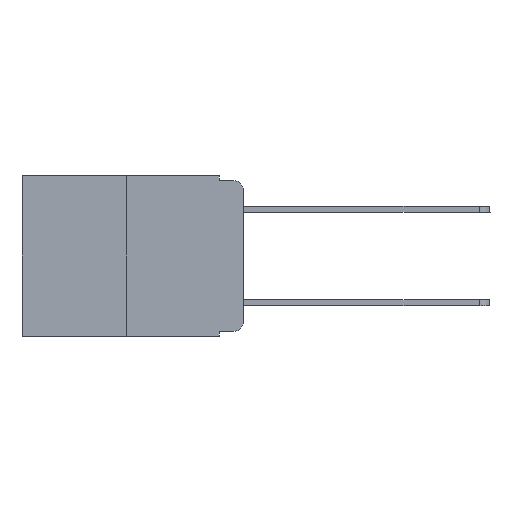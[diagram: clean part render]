
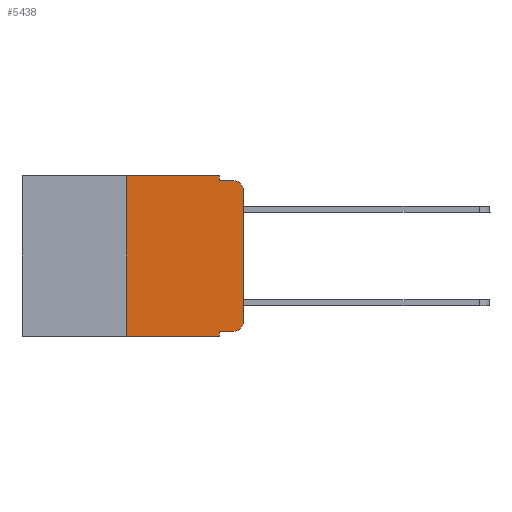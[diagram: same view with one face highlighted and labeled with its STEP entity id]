
A CAD part, left-side view. The second image highlights one B-rep face of the part: STEP entity #5438.
In plain terms, the highlighted planar face has unit normal (-1, 0, 0).
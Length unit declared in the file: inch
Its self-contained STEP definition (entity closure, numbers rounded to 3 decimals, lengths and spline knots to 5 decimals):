
#34 = CARTESIAN_POINT ( 'NONE',  ( 0., 0.25, -0.343 ) ) ;
#55 = EDGE_CURVE ( 'NONE', #1467, #11589, #5003, .T. ) ;
#94 = ORIENTED_EDGE ( 'NONE', *, *, #7449, .T. ) ;
#818 = LINE ( 'NONE', #9619, #1264 ) ;
#822 = CARTESIAN_POINT ( 'NONE',  ( 0., 0.473, 0. ) ) ;
#909 = ORIENTED_EDGE ( 'NONE', *, *, #7644, .T. ) ;
#1184 = LINE ( 'NONE', #5515, #7079 ) ;
#1203 = LINE ( 'NONE', #2210, #11564 ) ;
#1264 = VECTOR ( 'NONE', #2092, 39.37008 ) ;
#1420 = AXIS2_PLACEMENT_3D ( 'NONE', #4175, #13900, #6305 ) ;
#1427 = EDGE_CURVE ( 'NONE', #5306, #13583, #5239, .T. ) ;
#1467 = VERTEX_POINT ( 'NONE', #11957 ) ;
#1796 = DIRECTION ( 'NONE',  ( 0., 0., -1. ) ) ;
#1996 = VECTOR ( 'NONE', #12191, 39.37008 ) ;
#2050 = DIRECTION ( 'NONE',  ( 0., 0., -1. ) ) ;
#2092 = DIRECTION ( 'NONE',  ( 0., -1., 0. ) ) ;
#2210 = CARTESIAN_POINT ( 'NONE',  ( 0., 0., 0. ) ) ;
#2395 = EDGE_CURVE ( 'NONE', #11589, #13583, #818, .T. ) ;
#2417 = EDGE_LOOP ( 'NONE', ( #6809, #4321, #7530, #4868, #9445, #11373, #909, #8463, #12309, #94 ) ) ;
#2579 = VERTEX_POINT ( 'NONE', #34 ) ;
#3213 = CARTESIAN_POINT ( 'NONE',  ( 0., 0., -0.313 ) ) ;
#3253 = VERTEX_POINT ( 'NONE', #3801 ) ;
#3503 = CARTESIAN_POINT ( 'NONE',  ( 0., 0., -0.03 ) ) ;
#3801 = CARTESIAN_POINT ( 'NONE',  ( 0., 0.051, -0.333 ) ) ;
#4073 = EDGE_CURVE ( 'NONE', #3253, #7361, #7893, .T. ) ;
#4175 = CARTESIAN_POINT ( 'NONE',  ( 0., 0.02, -0.313 ) ) ;
#4321 = ORIENTED_EDGE ( 'NONE', *, *, #1427, .T. ) ;
#4738 = CARTESIAN_POINT ( 'NONE',  ( 0., 0.051, -0.333 ) ) ;
#4868 = ORIENTED_EDGE ( 'NONE', *, *, #55, .F. ) ;
#5003 = LINE ( 'NONE', #10753, #5395 ) ;
#5228 = DIRECTION ( 'NONE',  ( -1., 0., 0. ) ) ;
#5239 = CIRCLE ( 'NONE', #12024, 0.02 ) ;
#5306 = VERTEX_POINT ( 'NONE', #3503 ) ;
#5395 = VECTOR ( 'NONE', #13682, 39.37008 ) ;
#5438 = ADVANCED_FACE ( 'NONE', ( #8261 ), #10230, .F. ) ;
#5470 = AXIS2_PLACEMENT_3D ( 'NONE', #822, #6115, #8333 ) ;
#5472 = EDGE_CURVE ( 'NONE', #3253, #13927, #11492, .T. ) ;
#5515 = CARTESIAN_POINT ( 'NONE',  ( 0., 0.25, 0. ) ) ;
#5530 = DIRECTION ( 'NONE',  ( 0., -1., 0. ) ) ;
#5655 = LINE ( 'NONE', #12161, #10930 ) ;
#5964 = EDGE_CURVE ( 'NONE', #12203, #5306, #1203, .T. ) ;
#6115 = DIRECTION ( 'NONE',  ( 1., 0., 0. ) ) ;
#6299 = CARTESIAN_POINT ( 'NONE',  ( 0., 0.02, -0.03 ) ) ;
#6305 = DIRECTION ( 'NONE',  ( 0., 0., -1. ) ) ;
#6386 = CARTESIAN_POINT ( 'NONE',  ( 0., 0.051, -0.343 ) ) ;
#6809 = ORIENTED_EDGE ( 'NONE', *, *, #5964, .T. ) ;
#6831 = VECTOR ( 'NONE', #13072, 39.37008 ) ;
#7039 = CARTESIAN_POINT ( 'NONE',  ( 0., 0.051, 0. ) ) ;
#7079 = VECTOR ( 'NONE', #9843, 39.37008 ) ;
#7361 = VERTEX_POINT ( 'NONE', #11241 ) ;
#7415 = VERTEX_POINT ( 'NONE', #12594 ) ;
#7449 = EDGE_CURVE ( 'NONE', #7361, #12203, #7554, .T. ) ;
#7530 = ORIENTED_EDGE ( 'NONE', *, *, #2395, .F. ) ;
#7554 = CIRCLE ( 'NONE', #1420, 0.02 ) ;
#7644 = EDGE_CURVE ( 'NONE', #2579, #13927, #5655, .T. ) ;
#7883 = LINE ( 'NONE', #8946, #6831 ) ;
#7893 = LINE ( 'NONE', #4738, #1996 ) ;
#8261 = FACE_OUTER_BOUND ( 'NONE', #2417, .T. ) ;
#8333 = DIRECTION ( 'NONE',  ( 0., 0., -1. ) ) ;
#8463 = ORIENTED_EDGE ( 'NONE', *, *, #5472, .F. ) ;
#8787 = DIRECTION ( 'NONE',  ( 0., 0., 1. ) ) ;
#8946 = CARTESIAN_POINT ( 'NONE',  ( 0., 0.473, 0. ) ) ;
#9262 = EDGE_CURVE ( 'NONE', #2579, #7415, #1184, .T. ) ;
#9445 = ORIENTED_EDGE ( 'NONE', *, *, #12260, .F. ) ;
#9619 = CARTESIAN_POINT ( 'NONE',  ( 0., 0.051, -0.01 ) ) ;
#9843 = DIRECTION ( 'NONE',  ( 0., 0., 1. ) ) ;
#10230 = PLANE ( 'NONE',  #5470 ) ;
#10753 = CARTESIAN_POINT ( 'NONE',  ( 0., 0.051, 0. ) ) ;
#10930 = VECTOR ( 'NONE', #5530, 39.37008 ) ;
#11241 = CARTESIAN_POINT ( 'NONE',  ( 0., 0.02, -0.333 ) ) ;
#11373 = ORIENTED_EDGE ( 'NONE', *, *, #9262, .F. ) ;
#11492 = LINE ( 'NONE', #7039, #11557 ) ;
#11557 = VECTOR ( 'NONE', #1796, 39.37008 ) ;
#11564 = VECTOR ( 'NONE', #8787, 39.37008 ) ;
#11589 = VERTEX_POINT ( 'NONE', #12631 ) ;
#11957 = CARTESIAN_POINT ( 'NONE',  ( 0., 0.051, 0. ) ) ;
#12024 = AXIS2_PLACEMENT_3D ( 'NONE', #6299, #5228, #2050 ) ;
#12161 = CARTESIAN_POINT ( 'NONE',  ( 0., 0.473, -0.343 ) ) ;
#12191 = DIRECTION ( 'NONE',  ( 0., -1., 0. ) ) ;
#12203 = VERTEX_POINT ( 'NONE', #3213 ) ;
#12254 = CARTESIAN_POINT ( 'NONE',  ( 0., 0.02, -0.01 ) ) ;
#12260 = EDGE_CURVE ( 'NONE', #7415, #1467, #7883, .T. ) ;
#12309 = ORIENTED_EDGE ( 'NONE', *, *, #4073, .T. ) ;
#12594 = CARTESIAN_POINT ( 'NONE',  ( 0., 0.25, 0. ) ) ;
#12631 = CARTESIAN_POINT ( 'NONE',  ( 0., 0.051, -0.01 ) ) ;
#13072 = DIRECTION ( 'NONE',  ( 0., -1., 0. ) ) ;
#13583 = VERTEX_POINT ( 'NONE', #12254 ) ;
#13682 = DIRECTION ( 'NONE',  ( 0., 0., -1. ) ) ;
#13900 = DIRECTION ( 'NONE',  ( -1., 0., 0. ) ) ;
#13927 = VERTEX_POINT ( 'NONE', #6386 ) ;
